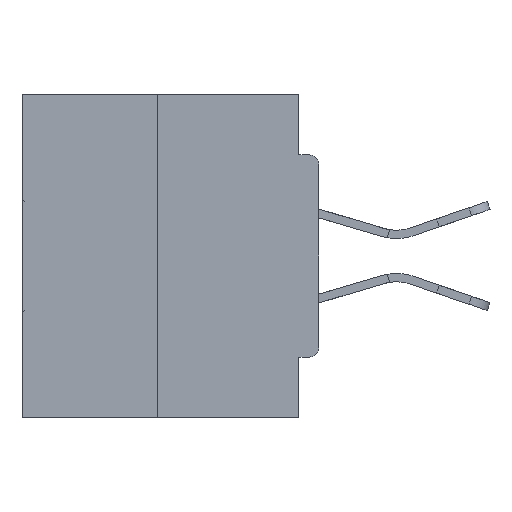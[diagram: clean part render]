
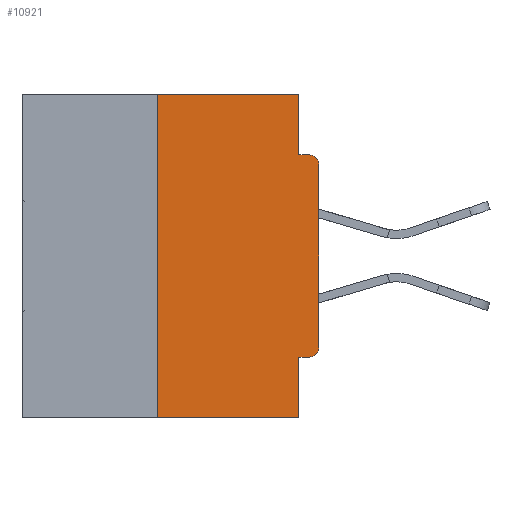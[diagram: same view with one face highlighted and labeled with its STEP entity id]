
A CAD part, left-side view. The second image highlights one B-rep face of the part: STEP entity #10921.
In plain terms, the highlighted planar face has unit normal (-1, 0, 0).
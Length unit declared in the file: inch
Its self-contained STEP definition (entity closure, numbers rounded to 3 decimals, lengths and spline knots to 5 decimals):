
#37 = EDGE_LOOP ( 'NONE', ( #2485, #21853, #38836, #22363, #76, #38537, #16940, #7816, #25405, #11033 ) ) ;
#76 = ORIENTED_EDGE ( 'NONE', *, *, #18531, .F. ) ;
#829 = LINE ( 'NONE', #2210, #12708 ) ;
#1753 = AXIS2_PLACEMENT_3D ( 'NONE', #22908, #33268, #13381 ) ;
#2210 = CARTESIAN_POINT ( 'NONE',  ( 0., 0., -0.0935 ) ) ;
#2485 = ORIENTED_EDGE ( 'NONE', *, *, #3846, .F. ) ;
#3846 = EDGE_CURVE ( 'NONE', #15119, #18804, #25241, .T. ) ;
#4240 = CARTESIAN_POINT ( 'NONE',  ( 0., 0.25, 0. ) ) ;
#4244 = VERTEX_POINT ( 'NONE', #19891 ) ;
#4966 = FACE_OUTER_BOUND ( 'NONE', #37, .T. ) ;
#6568 = CARTESIAN_POINT ( 'NONE',  ( 0., 0.46, 0. ) ) ;
#7816 = ORIENTED_EDGE ( 'NONE', *, *, #21821, .T. ) ;
#8048 = CARTESIAN_POINT ( 'NONE',  ( 0., 0.46, 0. ) ) ;
#8478 = DIRECTION ( 'NONE',  ( 0., 0., -1. ) ) ;
#9094 = CARTESIAN_POINT ( 'NONE',  ( 0., 0.015, -0.0935 ) ) ;
#9519 = CARTESIAN_POINT ( 'NONE',  ( 0., 0., -0.1085 ) ) ;
#9632 = CARTESIAN_POINT ( 'NONE',  ( 0., 0.25, 0. ) ) ;
#9952 = LINE ( 'NONE', #36759, #38278 ) ;
#10921 = ADVANCED_FACE ( 'NONE', ( #4966 ), #21595, .F. ) ;
#11033 = ORIENTED_EDGE ( 'NONE', *, *, #19736, .F. ) ;
#11738 = VERTEX_POINT ( 'NONE', #25071 ) ;
#12438 = DIRECTION ( 'NONE',  ( 0., -1., 0. ) ) ;
#12626 = CARTESIAN_POINT ( 'NONE',  ( 0., 0.031, -0.0935 ) ) ;
#12708 = VECTOR ( 'NONE', #12438, 39.37008 ) ;
#13381 = DIRECTION ( 'NONE',  ( 0., 0., -1. ) ) ;
#13797 = EDGE_CURVE ( 'NONE', #32740, #26319, #22660, .T. ) ;
#15119 = VERTEX_POINT ( 'NONE', #9632 ) ;
#15195 = VECTOR ( 'NONE', #24657, 39.37008 ) ;
#15991 = CARTESIAN_POINT ( 'NONE',  ( 0., 0.031, -0.5 ) ) ;
#16192 = EDGE_CURVE ( 'NONE', #32740, #15119, #27538, .T. ) ;
#16659 = VECTOR ( 'NONE', #35578, 39.37008 ) ;
#16940 = ORIENTED_EDGE ( 'NONE', *, *, #20556, .T. ) ;
#17248 = VERTEX_POINT ( 'NONE', #9094 ) ;
#17677 = CARTESIAN_POINT ( 'NONE',  ( 0., 0.031, -0.5 ) ) ;
#18048 = AXIS2_PLACEMENT_3D ( 'NONE', #8048, #40866, #8478 ) ;
#18531 = EDGE_CURVE ( 'NONE', #4244, #11738, #26332, .T. ) ;
#18804 = VERTEX_POINT ( 'NONE', #19053 ) ;
#19053 = CARTESIAN_POINT ( 'NONE',  ( 0., 0.031, 0. ) ) ;
#19194 = DIRECTION ( 'NONE',  ( -1., 0., 0. ) ) ;
#19370 = CARTESIAN_POINT ( 'NONE',  ( 0., 0., -0.3915 ) ) ;
#19736 = EDGE_CURVE ( 'NONE', #18804, #37370, #26025, .T. ) ;
#19891 = CARTESIAN_POINT ( 'NONE',  ( 0., 0.015, -0.4065 ) ) ;
#20208 = CARTESIAN_POINT ( 'NONE',  ( 0., 0.25, -0.5 ) ) ;
#20556 = EDGE_CURVE ( 'NONE', #28610, #33279, #9952, .T. ) ;
#20739 = EDGE_CURVE ( 'NONE', #11738, #26319, #30576, .T. ) ;
#21595 = PLANE ( 'NONE',  #18048 ) ;
#21821 = EDGE_CURVE ( 'NONE', #33279, #17248, #24335, .T. ) ;
#21853 = ORIENTED_EDGE ( 'NONE', *, *, #16192, .F. ) ;
#22231 = CARTESIAN_POINT ( 'NONE',  ( 0., 0.015, -0.3915 ) ) ;
#22285 = CARTESIAN_POINT ( 'NONE',  ( 0., 0., -0.4065 ) ) ;
#22363 = ORIENTED_EDGE ( 'NONE', *, *, #20739, .F. ) ;
#22504 = AXIS2_PLACEMENT_3D ( 'NONE', #22231, #19194, #25394 ) ;
#22660 = LINE ( 'NONE', #37559, #26261 ) ;
#22908 = CARTESIAN_POINT ( 'NONE',  ( 0., 0.015, -0.1085 ) ) ;
#24226 = CARTESIAN_POINT ( 'NONE',  ( 0., 0.031, 0. ) ) ;
#24335 = CIRCLE ( 'NONE', #1753, 0.015 ) ;
#24657 = DIRECTION ( 'NONE',  ( 0., 0., -1. ) ) ;
#25071 = CARTESIAN_POINT ( 'NONE',  ( 0., 0.031, -0.4065 ) ) ;
#25241 = LINE ( 'NONE', #6568, #40675 ) ;
#25394 = DIRECTION ( 'NONE',  ( 0., 0., -1. ) ) ;
#25405 = ORIENTED_EDGE ( 'NONE', *, *, #35510, .F. ) ;
#26025 = LINE ( 'NONE', #24226, #15195 ) ;
#26061 = DIRECTION ( 'NONE',  ( 0., -1., 0. ) ) ;
#26261 = VECTOR ( 'NONE', #34941, 39.37008 ) ;
#26319 = VERTEX_POINT ( 'NONE', #17677 ) ;
#26332 = LINE ( 'NONE', #22285, #28883 ) ;
#27538 = LINE ( 'NONE', #4240, #38858 ) ;
#27666 = CIRCLE ( 'NONE', #22504, 0.015 ) ;
#28610 = VERTEX_POINT ( 'NONE', #19370 ) ;
#28883 = VECTOR ( 'NONE', #30760, 39.37008 ) ;
#30295 = DIRECTION ( 'NONE',  ( 0., 0., 1. ) ) ;
#30576 = LINE ( 'NONE', #15991, #16659 ) ;
#30760 = DIRECTION ( 'NONE',  ( 0., 1., 0. ) ) ;
#32740 = VERTEX_POINT ( 'NONE', #20208 ) ;
#33268 = DIRECTION ( 'NONE',  ( -1., 0., 0. ) ) ;
#33279 = VERTEX_POINT ( 'NONE', #9519 ) ;
#34941 = DIRECTION ( 'NONE',  ( 0., -1., 0. ) ) ;
#35510 = EDGE_CURVE ( 'NONE', #37370, #17248, #829, .T. ) ;
#35578 = DIRECTION ( 'NONE',  ( 0., 0., -1. ) ) ;
#36427 = EDGE_CURVE ( 'NONE', #4244, #28610, #27666, .T. ) ;
#36759 = CARTESIAN_POINT ( 'NONE',  ( 0., 0., 0. ) ) ;
#37370 = VERTEX_POINT ( 'NONE', #12626 ) ;
#37559 = CARTESIAN_POINT ( 'NONE',  ( 0., 0.46, -0.5 ) ) ;
#38278 = VECTOR ( 'NONE', #30295, 39.37008 ) ;
#38537 = ORIENTED_EDGE ( 'NONE', *, *, #36427, .T. ) ;
#38836 = ORIENTED_EDGE ( 'NONE', *, *, #13797, .T. ) ;
#38858 = VECTOR ( 'NONE', #40630, 39.37008 ) ;
#40630 = DIRECTION ( 'NONE',  ( 0., 0., 1. ) ) ;
#40675 = VECTOR ( 'NONE', #26061, 39.37008 ) ;
#40866 = DIRECTION ( 'NONE',  ( 1., 0., 0. ) ) ;
